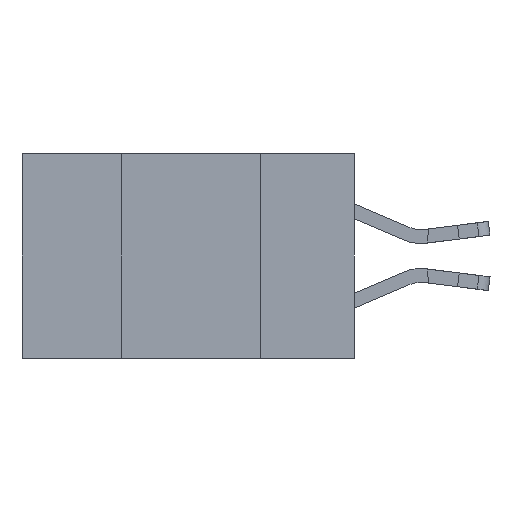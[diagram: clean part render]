
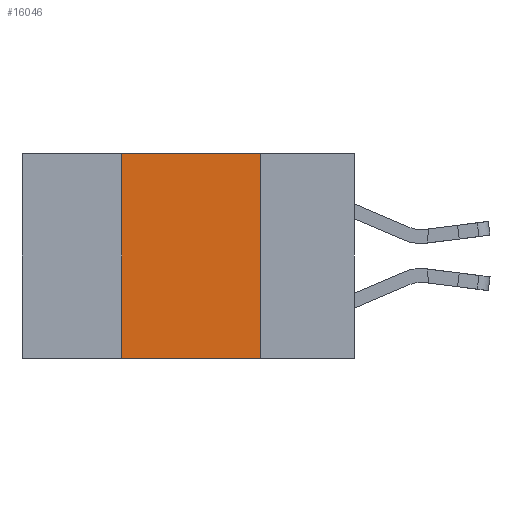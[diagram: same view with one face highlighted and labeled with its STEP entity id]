
A CAD part, left-side view. The second image highlights one B-rep face of the part: STEP entity #16046.
In plain terms, the highlighted planar face has unit normal (-1, 0, 0).
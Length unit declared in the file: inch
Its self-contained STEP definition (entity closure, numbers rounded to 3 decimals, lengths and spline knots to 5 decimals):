
#195 = AXIS2_PLACEMENT_3D ( 'NONE', #9383, #10739, #2499 ) ;
#1089 = EDGE_CURVE ( 'NONE', #3350, #2292, #1549, .T. ) ;
#1549 = LINE ( 'NONE', #2394, #8534 ) ;
#2292 = VERTEX_POINT ( 'NONE', #12891 ) ;
#2394 = CARTESIAN_POINT ( 'NONE',  ( 0., 0.17, -0.37 ) ) ;
#2427 = EDGE_CURVE ( 'NONE', #10116, #3350, #2892, .T. ) ;
#2499 = DIRECTION ( 'NONE',  ( 0., 0., -1. ) ) ;
#2892 = LINE ( 'NONE', #10862, #9773 ) ;
#3350 = VERTEX_POINT ( 'NONE', #14729 ) ;
#4287 = VECTOR ( 'NONE', #8599, 39.37008 ) ;
#7201 = ORIENTED_EDGE ( 'NONE', *, *, #16191, .T. ) ;
#7894 = LINE ( 'NONE', #16589, #4287 ) ;
#8534 = VECTOR ( 'NONE', #14583, 39.37008 ) ;
#8599 = DIRECTION ( 'NONE',  ( 0., -1., 0. ) ) ;
#9005 = CARTESIAN_POINT ( 'NONE',  ( 0., 0.42, -0.37 ) ) ;
#9383 = CARTESIAN_POINT ( 'NONE',  ( 0., 0.6, 0. ) ) ;
#9773 = VECTOR ( 'NONE', #11003, 39.37008 ) ;
#10116 = VERTEX_POINT ( 'NONE', #17632 ) ;
#10304 = VECTOR ( 'NONE', #17005, 39.37008 ) ;
#10739 = DIRECTION ( 'NONE',  ( 1., 0., 0. ) ) ;
#10766 = EDGE_LOOP ( 'NONE', ( #10803, #16811, #15959, #7201 ) ) ;
#10803 = ORIENTED_EDGE ( 'NONE', *, *, #1089, .F. ) ;
#10862 = CARTESIAN_POINT ( 'NONE',  ( 0., 0.6, 0. ) ) ;
#11003 = DIRECTION ( 'NONE',  ( 0., -1., 0. ) ) ;
#12794 = CARTESIAN_POINT ( 'NONE',  ( 0., 0.42, -0.37 ) ) ;
#12891 = CARTESIAN_POINT ( 'NONE',  ( 0., 0.17, -0.37 ) ) ;
#13821 = LINE ( 'NONE', #9005, #10304 ) ;
#14423 = EDGE_CURVE ( 'NONE', #17015, #10116, #13821, .T. ) ;
#14583 = DIRECTION ( 'NONE',  ( 0., 0., -1. ) ) ;
#14729 = CARTESIAN_POINT ( 'NONE',  ( 0., 0.17, 0. ) ) ;
#15959 = ORIENTED_EDGE ( 'NONE', *, *, #14423, .F. ) ;
#16046 = ADVANCED_FACE ( 'NONE', ( #17107 ), #17366, .F. ) ;
#16191 = EDGE_CURVE ( 'NONE', #17015, #2292, #7894, .T. ) ;
#16589 = CARTESIAN_POINT ( 'NONE',  ( 0., 0.6, -0.37 ) ) ;
#16811 = ORIENTED_EDGE ( 'NONE', *, *, #2427, .F. ) ;
#17005 = DIRECTION ( 'NONE',  ( 0., 0., 1. ) ) ;
#17015 = VERTEX_POINT ( 'NONE', #12794 ) ;
#17107 = FACE_OUTER_BOUND ( 'NONE', #10766, .T. ) ;
#17366 = PLANE ( 'NONE',  #195 ) ;
#17632 = CARTESIAN_POINT ( 'NONE',  ( 0., 0.42, 0. ) ) ;
